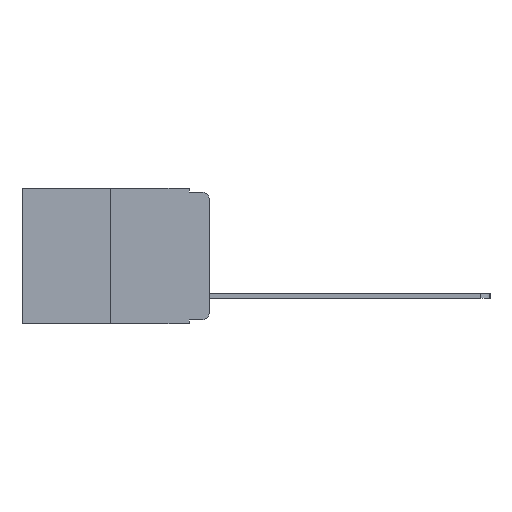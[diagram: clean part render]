
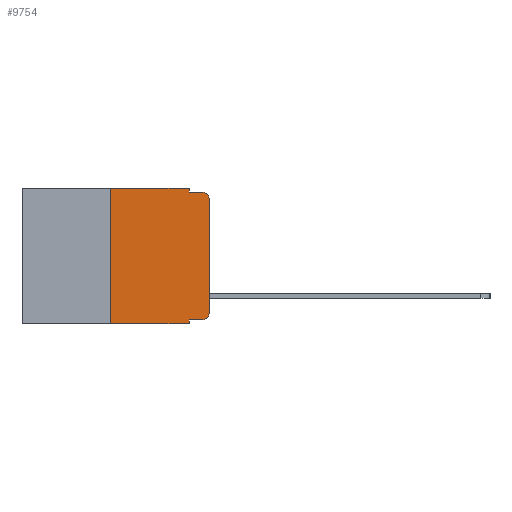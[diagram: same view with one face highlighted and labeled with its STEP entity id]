
A CAD part, left-side view. The second image highlights one B-rep face of the part: STEP entity #9754.
In plain terms, the highlighted planar face has unit normal (-1, 0, 0).
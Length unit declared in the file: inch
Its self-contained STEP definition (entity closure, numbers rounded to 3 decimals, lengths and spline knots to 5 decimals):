
#370 = CARTESIAN_POINT ( 'NONE',  ( 0., 0.051, -0.333 ) ) ;
#499 = DIRECTION ( 'NONE',  ( 0., 0., -1. ) ) ;
#518 = CARTESIAN_POINT ( 'NONE',  ( 0., 0., -0.03 ) ) ;
#1411 = DIRECTION ( 'NONE',  ( -1., 0., 0. ) ) ;
#1516 = EDGE_CURVE ( 'NONE', #3495, #6535, #6808, .T. ) ;
#1691 = EDGE_CURVE ( 'NONE', #16725, #7424, #3372, .T. ) ;
#1824 = VERTEX_POINT ( 'NONE', #10514 ) ;
#1898 = VERTEX_POINT ( 'NONE', #518 ) ;
#1901 = LINE ( 'NONE', #8376, #5524 ) ;
#2087 = CARTESIAN_POINT ( 'NONE',  ( 0., 0.473, -0.343 ) ) ;
#2214 = PLANE ( 'NONE',  #15671 ) ;
#2546 = EDGE_CURVE ( 'NONE', #11642, #16725, #12319, .T. ) ;
#3372 = LINE ( 'NONE', #7089, #15739 ) ;
#3434 = ORIENTED_EDGE ( 'NONE', *, *, #1516, .F. ) ;
#3495 = VERTEX_POINT ( 'NONE', #370 ) ;
#4420 = ORIENTED_EDGE ( 'NONE', *, *, #18792, .T. ) ;
#4449 = EDGE_LOOP ( 'NONE', ( #7211, #12610, #9190, #16940, #17395, #6139, #11037, #3434, #4420, #12405 ) ) ;
#4574 = LINE ( 'NONE', #16305, #15945 ) ;
#4610 = EDGE_CURVE ( 'NONE', #7424, #8966, #10305, .T. ) ;
#4895 = FACE_OUTER_BOUND ( 'NONE', #4449, .T. ) ;
#4943 = CARTESIAN_POINT ( 'NONE',  ( 0., 0.051, -0.01 ) ) ;
#5327 = CARTESIAN_POINT ( 'NONE',  ( 0., 0.473, 0. ) ) ;
#5339 = DIRECTION ( 'NONE',  ( 0., 0., 1. ) ) ;
#5524 = VECTOR ( 'NONE', #5339, 39.37008 ) ;
#5669 = EDGE_CURVE ( 'NONE', #8966, #16113, #12557, .T. ) ;
#5917 = CARTESIAN_POINT ( 'NONE',  ( 0., 0.25, -0.343 ) ) ;
#6120 = VECTOR ( 'NONE', #499, 39.37008 ) ;
#6139 = ORIENTED_EDGE ( 'NONE', *, *, #2546, .F. ) ;
#6535 = VERTEX_POINT ( 'NONE', #10516 ) ;
#6742 = DIRECTION ( 'NONE',  ( 0., -1., 0. ) ) ;
#6808 = LINE ( 'NONE', #11528, #17569 ) ;
#6867 = DIRECTION ( 'NONE',  ( 0., 0., -1. ) ) ;
#7042 = DIRECTION ( 'NONE',  ( 0., -1., 0. ) ) ;
#7089 = CARTESIAN_POINT ( 'NONE',  ( 0., 0.473, 0. ) ) ;
#7211 = ORIENTED_EDGE ( 'NONE', *, *, #12635, .T. ) ;
#7424 = VERTEX_POINT ( 'NONE', #17014 ) ;
#7694 = EDGE_CURVE ( 'NONE', #1898, #16113, #16567, .T. ) ;
#8177 = VECTOR ( 'NONE', #14905, 39.37008 ) ;
#8376 = CARTESIAN_POINT ( 'NONE',  ( 0., 0., 0. ) ) ;
#8527 = VERTEX_POINT ( 'NONE', #15182 ) ;
#8749 = CARTESIAN_POINT ( 'NONE',  ( 0., 0.051, -0.01 ) ) ;
#8915 = CARTESIAN_POINT ( 'NONE',  ( 0., 0.02, -0.03 ) ) ;
#8966 = VERTEX_POINT ( 'NONE', #4943 ) ;
#9190 = ORIENTED_EDGE ( 'NONE', *, *, #5669, .F. ) ;
#9754 = ADVANCED_FACE ( 'NONE', ( #4895 ), #2214, .F. ) ;
#10305 = LINE ( 'NONE', #17651, #6120 ) ;
#10410 = DIRECTION ( 'NONE',  ( 0., 0., -1. ) ) ;
#10514 = CARTESIAN_POINT ( 'NONE',  ( 0., 0.02, -0.333 ) ) ;
#10516 = CARTESIAN_POINT ( 'NONE',  ( 0., 0.051, -0.343 ) ) ;
#10530 = CARTESIAN_POINT ( 'NONE',  ( 0., 0.02, -0.313 ) ) ;
#11037 = ORIENTED_EDGE ( 'NONE', *, *, #11449, .T. ) ;
#11449 = EDGE_CURVE ( 'NONE', #11642, #6535, #11849, .T. ) ;
#11528 = CARTESIAN_POINT ( 'NONE',  ( 0., 0.051, 0. ) ) ;
#11642 = VERTEX_POINT ( 'NONE', #5917 ) ;
#11849 = LINE ( 'NONE', #2087, #19063 ) ;
#11985 = DIRECTION ( 'NONE',  ( 0., 0., -1. ) ) ;
#12117 = DIRECTION ( 'NONE',  ( 0., 0., 1. ) ) ;
#12319 = LINE ( 'NONE', #17204, #18625 ) ;
#12405 = ORIENTED_EDGE ( 'NONE', *, *, #17857, .T. ) ;
#12557 = LINE ( 'NONE', #8749, #8177 ) ;
#12610 = ORIENTED_EDGE ( 'NONE', *, *, #7694, .T. ) ;
#12635 = EDGE_CURVE ( 'NONE', #8527, #1898, #1901, .T. ) ;
#12804 = CIRCLE ( 'NONE', #18445, 0.02 ) ;
#12989 = DIRECTION ( 'NONE',  ( 0., 0., -1. ) ) ;
#14905 = DIRECTION ( 'NONE',  ( 0., -1., 0. ) ) ;
#15182 = CARTESIAN_POINT ( 'NONE',  ( 0., 0., -0.313 ) ) ;
#15641 = DIRECTION ( 'NONE',  ( 1., 0., 0. ) ) ;
#15671 = AXIS2_PLACEMENT_3D ( 'NONE', #5327, #15641, #6867 ) ;
#15739 = VECTOR ( 'NONE', #7042, 39.37008 ) ;
#15945 = VECTOR ( 'NONE', #17756, 39.37008 ) ;
#16113 = VERTEX_POINT ( 'NONE', #16810 ) ;
#16172 = AXIS2_PLACEMENT_3D ( 'NONE', #8915, #19047, #10410 ) ;
#16305 = CARTESIAN_POINT ( 'NONE',  ( 0., 0.051, -0.333 ) ) ;
#16567 = CIRCLE ( 'NONE', #16172, 0.02 ) ;
#16725 = VERTEX_POINT ( 'NONE', #18240 ) ;
#16810 = CARTESIAN_POINT ( 'NONE',  ( 0., 0.02, -0.01 ) ) ;
#16940 = ORIENTED_EDGE ( 'NONE', *, *, #4610, .F. ) ;
#17014 = CARTESIAN_POINT ( 'NONE',  ( 0., 0.051, 0. ) ) ;
#17204 = CARTESIAN_POINT ( 'NONE',  ( 0., 0.25, 0. ) ) ;
#17395 = ORIENTED_EDGE ( 'NONE', *, *, #1691, .F. ) ;
#17569 = VECTOR ( 'NONE', #12989, 39.37008 ) ;
#17651 = CARTESIAN_POINT ( 'NONE',  ( 0., 0.051, 0. ) ) ;
#17756 = DIRECTION ( 'NONE',  ( 0., -1., 0. ) ) ;
#17857 = EDGE_CURVE ( 'NONE', #1824, #8527, #12804, .T. ) ;
#18240 = CARTESIAN_POINT ( 'NONE',  ( 0., 0.25, 0. ) ) ;
#18445 = AXIS2_PLACEMENT_3D ( 'NONE', #10530, #1411, #11985 ) ;
#18625 = VECTOR ( 'NONE', #12117, 39.37008 ) ;
#18792 = EDGE_CURVE ( 'NONE', #3495, #1824, #4574, .T. ) ;
#19047 = DIRECTION ( 'NONE',  ( -1., 0., 0. ) ) ;
#19063 = VECTOR ( 'NONE', #6742, 39.37008 ) ;
